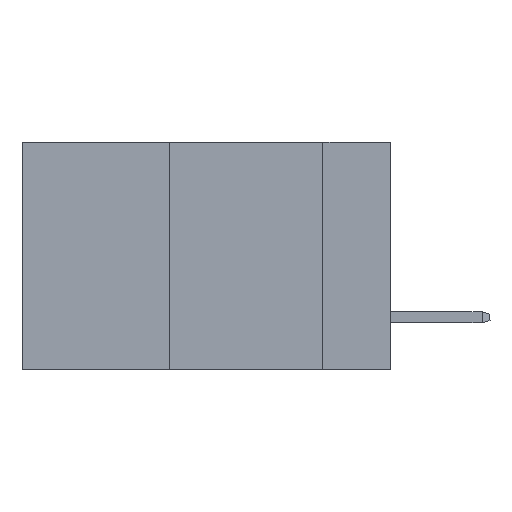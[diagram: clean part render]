
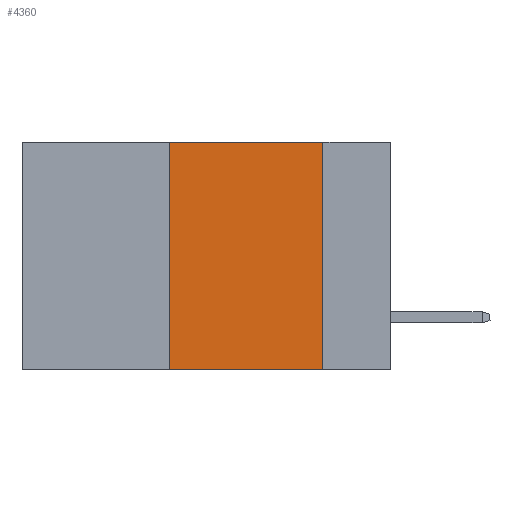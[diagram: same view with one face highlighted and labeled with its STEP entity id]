
A CAD part, left-side view. The second image highlights one B-rep face of the part: STEP entity #4360.
In plain terms, the highlighted planar face has unit normal (-1, 0, 0).
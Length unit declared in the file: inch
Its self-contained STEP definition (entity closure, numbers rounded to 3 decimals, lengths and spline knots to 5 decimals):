
#205 = ORIENTED_EDGE ( 'NONE', *, *, #6815, .F. ) ;
#234 = DIRECTION ( 'NONE',  ( 1., 0., 0. ) ) ;
#245 = ORIENTED_EDGE ( 'NONE', *, *, #6208, .F. ) ;
#274 = CARTESIAN_POINT ( 'NONE',  ( 0., 0.6, -0.37 ) ) ;
#349 = DIRECTION ( 'NONE',  ( 0., 0., -1. ) ) ;
#496 = ORIENTED_EDGE ( 'NONE', *, *, #15918, .F. ) ;
#516 = ORIENTED_EDGE ( 'NONE', *, *, #9975, .T. ) ;
#916 = DIRECTION ( 'NONE',  ( 0., 0., -1. ) ) ;
#1390 = PLANE ( 'NONE',  #10176 ) ;
#2359 = VECTOR ( 'NONE', #3692, 39.37008 ) ;
#2382 = CARTESIAN_POINT ( 'NONE',  ( 0., 0.11, -0.37 ) ) ;
#2556 = LINE ( 'NONE', #17135, #9601 ) ;
#3692 = DIRECTION ( 'NONE',  ( 0., -1., 0. ) ) ;
#3907 = CARTESIAN_POINT ( 'NONE',  ( 0., 0.6, 0. ) ) ;
#4360 = ADVANCED_FACE ( 'NONE', ( #5882 ), #1390, .F. ) ;
#4867 = DIRECTION ( 'NONE',  ( 0., -1., 0. ) ) ;
#5882 = FACE_OUTER_BOUND ( 'NONE', #11535, .T. ) ;
#6208 = EDGE_CURVE ( 'NONE', #13014, #12168, #6649, .T. ) ;
#6649 = LINE ( 'NONE', #3907, #2359 ) ;
#6815 = EDGE_CURVE ( 'NONE', #12168, #11295, #2556, .T. ) ;
#7895 = VERTEX_POINT ( 'NONE', #9048 ) ;
#8462 = LINE ( 'NONE', #274, #17483 ) ;
#8769 = LINE ( 'NONE', #9087, #14834 ) ;
#9048 = CARTESIAN_POINT ( 'NONE',  ( 0., 0.36, -0.37 ) ) ;
#9087 = CARTESIAN_POINT ( 'NONE',  ( 0., 0.36, 0. ) ) ;
#9601 = VECTOR ( 'NONE', #916, 39.37008 ) ;
#9975 = EDGE_CURVE ( 'NONE', #7895, #11295, #8462, .T. ) ;
#10176 = AXIS2_PLACEMENT_3D ( 'NONE', #17508, #234, #349 ) ;
#10830 = CARTESIAN_POINT ( 'NONE',  ( 0., 0.36, 0. ) ) ;
#11220 = CARTESIAN_POINT ( 'NONE',  ( 0., 0.11, 0. ) ) ;
#11295 = VERTEX_POINT ( 'NONE', #2382 ) ;
#11535 = EDGE_LOOP ( 'NONE', ( #205, #245, #496, #516 ) ) ;
#12168 = VERTEX_POINT ( 'NONE', #11220 ) ;
#13014 = VERTEX_POINT ( 'NONE', #10830 ) ;
#14834 = VECTOR ( 'NONE', #15514, 39.37008 ) ;
#15514 = DIRECTION ( 'NONE',  ( 0., 0., 1. ) ) ;
#15918 = EDGE_CURVE ( 'NONE', #7895, #13014, #8769, .T. ) ;
#17135 = CARTESIAN_POINT ( 'NONE',  ( 0., 0.11, 0. ) ) ;
#17483 = VECTOR ( 'NONE', #4867, 39.37008 ) ;
#17508 = CARTESIAN_POINT ( 'NONE',  ( 0., 0.6, 0. ) ) ;
